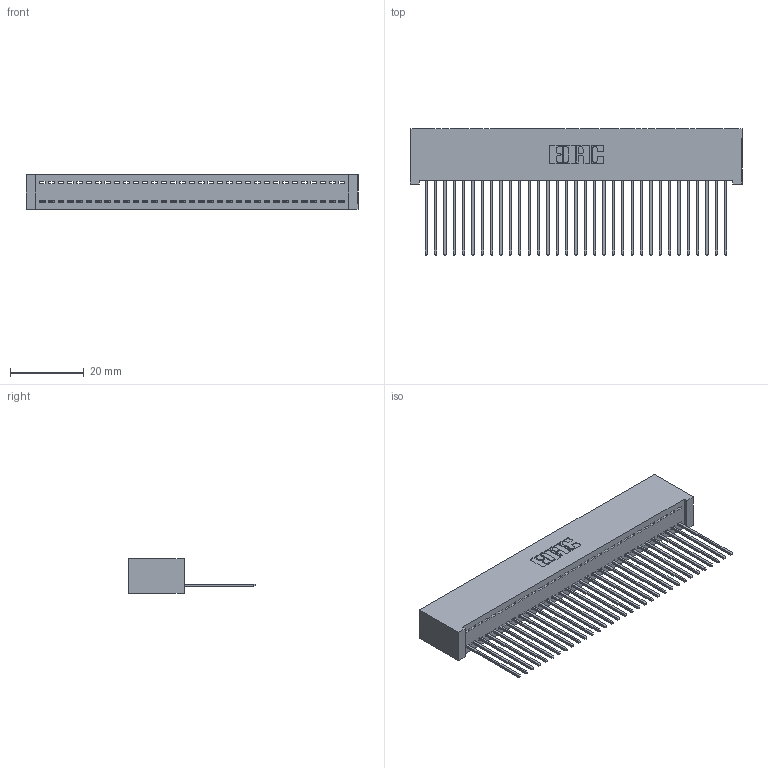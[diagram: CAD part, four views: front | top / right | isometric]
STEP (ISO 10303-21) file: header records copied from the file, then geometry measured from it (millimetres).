
FILE_DESCRIPTION (( 'STEP AP203' ), '1' );
FILE_NAME ('342-033-541-101.STEP', '2019-10-02T11:41:54', ( '' ), ( '' ), 'SwSTEP 2.0', 'SolidWorks 2016', '' );
FILE_SCHEMA (( 'CONFIG_CONTROL_DESIGN' ));
Length unit declared in the file: inch
Products named in the file (3): 342 Part_Lugless; 345-292-001_345-293-141; 342-033-541-101
Assembly tree (34 placements, depth 2):
  342-033-541-101
    342 Part_Lugless
    345-292-001_345-293-141  x33
Bounding box: 90.07 x 34.3 x 9.4 mm (x, y, z)
Volume: 8381.9 mm3; surface area: 13083 mm2
Topology: 34 solids, 34 shells, 2016 faces, 6083 edges, 4010 vertices
Faces by surface type: plane 1448, cylinder 568
Entity records: 20947 total; most frequent: CARTESIAN_POINT 3621, ORIENTED_EDGE 3590, DIRECTION 3065, EDGE_CURVE 1795, LINE 1675, VECTOR 1675, VERTEX_POINT 1194, AXIS2_PLACEMENT_3D 695
